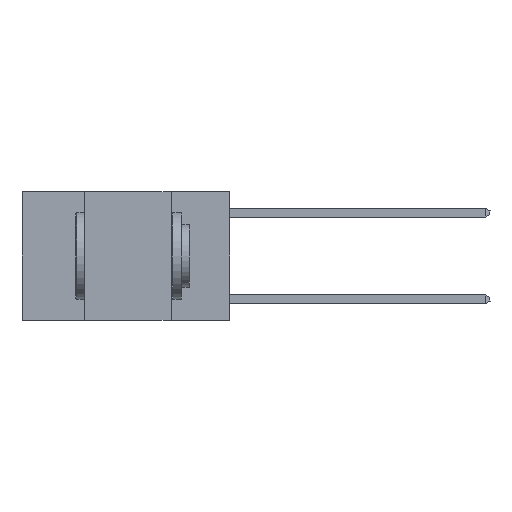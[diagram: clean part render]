
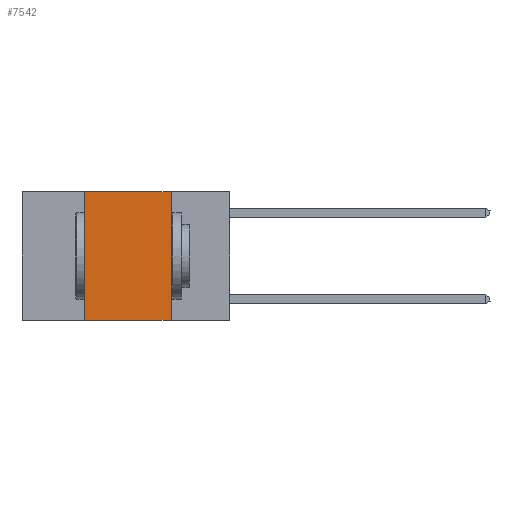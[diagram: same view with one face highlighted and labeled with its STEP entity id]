
A CAD part, left-side view. The second image highlights one B-rep face of the part: STEP entity #7542.
In plain terms, the highlighted planar face has unit normal (-1, 0, 0).
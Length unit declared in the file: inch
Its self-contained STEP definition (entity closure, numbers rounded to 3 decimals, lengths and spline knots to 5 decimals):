
#113 = VECTOR ( 'NONE', #1624, 39.37008 ) ;
#627 = CARTESIAN_POINT ( 'NONE',  ( 0., 0.17, -0.37 ) ) ;
#923 = LINE ( 'NONE', #9343, #113 ) ;
#1363 = CARTESIAN_POINT ( 'NONE',  ( 0., 0.17, 0. ) ) ;
#1624 = DIRECTION ( 'NONE',  ( 0., -1., 0. ) ) ;
#1688 = CARTESIAN_POINT ( 'NONE',  ( 0., 0.17, 0. ) ) ;
#1793 = EDGE_CURVE ( 'NONE', #8206, #6432, #9178, .T. ) ;
#1902 = ORIENTED_EDGE ( 'NONE', *, *, #1793, .T. ) ;
#1974 = EDGE_CURVE ( 'NONE', #2960, #7125, #923, .T. ) ;
#2921 = AXIS2_PLACEMENT_3D ( 'NONE', #8393, #4664, #3524 ) ;
#2960 = VERTEX_POINT ( 'NONE', #10185 ) ;
#3014 = VECTOR ( 'NONE', #9557, 39.37008 ) ;
#3524 = DIRECTION ( 'NONE',  ( 0., 0., -1. ) ) ;
#3707 = FACE_OUTER_BOUND ( 'NONE', #3755, .T. ) ;
#3755 = EDGE_LOOP ( 'NONE', ( #10235, #12126, #5466, #1902 ) ) ;
#3847 = LINE ( 'NONE', #5978, #5149 ) ;
#4406 = CARTESIAN_POINT ( 'NONE',  ( 0., 0.6, -0.37 ) ) ;
#4664 = DIRECTION ( 'NONE',  ( 1., 0., 0. ) ) ;
#5149 = VECTOR ( 'NONE', #8818, 39.37008 ) ;
#5466 = ORIENTED_EDGE ( 'NONE', *, *, #7581, .F. ) ;
#5848 = EDGE_CURVE ( 'NONE', #7125, #6432, #9276, .T. ) ;
#5978 = CARTESIAN_POINT ( 'NONE',  ( 0., 0.42, 0. ) ) ;
#6432 = VERTEX_POINT ( 'NONE', #627 ) ;
#7125 = VERTEX_POINT ( 'NONE', #1688 ) ;
#7542 = ADVANCED_FACE ( 'NONE', ( #3707 ), #9378, .F. ) ;
#7581 = EDGE_CURVE ( 'NONE', #8206, #2960, #3847, .T. ) ;
#8206 = VERTEX_POINT ( 'NONE', #11369 ) ;
#8393 = CARTESIAN_POINT ( 'NONE',  ( 0., 0.6, 0. ) ) ;
#8818 = DIRECTION ( 'NONE',  ( 0., 0., 1. ) ) ;
#9178 = LINE ( 'NONE', #4406, #3014 ) ;
#9276 = LINE ( 'NONE', #1363, #10137 ) ;
#9343 = CARTESIAN_POINT ( 'NONE',  ( 0., 0.6, 0. ) ) ;
#9378 = PLANE ( 'NONE',  #2921 ) ;
#9557 = DIRECTION ( 'NONE',  ( 0., -1., 0. ) ) ;
#10137 = VECTOR ( 'NONE', #11929, 39.37008 ) ;
#10185 = CARTESIAN_POINT ( 'NONE',  ( 0., 0.42, 0. ) ) ;
#10235 = ORIENTED_EDGE ( 'NONE', *, *, #5848, .F. ) ;
#11369 = CARTESIAN_POINT ( 'NONE',  ( 0., 0.42, -0.37 ) ) ;
#11929 = DIRECTION ( 'NONE',  ( 0., 0., -1. ) ) ;
#12126 = ORIENTED_EDGE ( 'NONE', *, *, #1974, .F. ) ;
